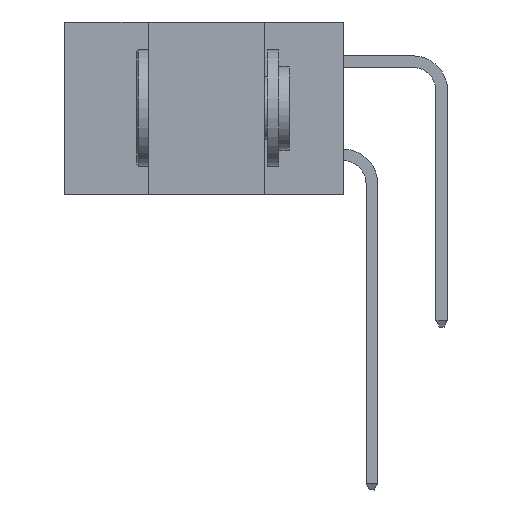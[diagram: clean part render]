
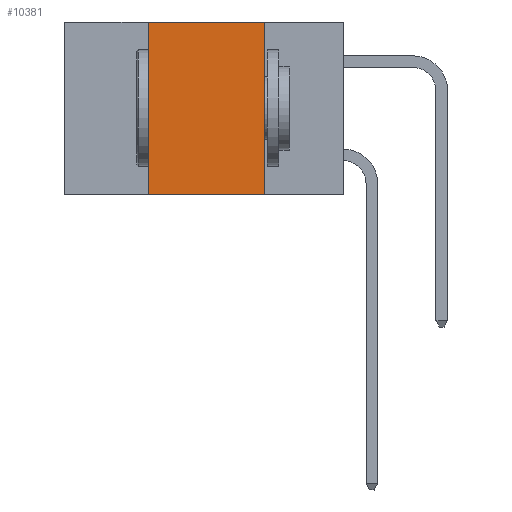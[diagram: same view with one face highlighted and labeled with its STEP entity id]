
A CAD part, left-side view. The second image highlights one B-rep face of the part: STEP entity #10381.
In plain terms, the highlighted planar face has unit normal (-1, 0, 0).
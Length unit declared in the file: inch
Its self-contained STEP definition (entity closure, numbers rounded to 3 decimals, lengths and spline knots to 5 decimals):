
#593 = CARTESIAN_POINT ( 'NONE',  ( 0., 0.17, -0.37 ) ) ;
#629 = ORIENTED_EDGE ( 'NONE', *, *, #6105, .F. ) ;
#1290 = CARTESIAN_POINT ( 'NONE',  ( 0., 0.6, 0. ) ) ;
#1818 = CARTESIAN_POINT ( 'NONE',  ( 0., 0.17, 0. ) ) ;
#2117 = EDGE_CURVE ( 'NONE', #4980, #7276, #3818, .T. ) ;
#2187 = EDGE_LOOP ( 'NONE', ( #10609, #5783, #629, #2998 ) ) ;
#2216 = CARTESIAN_POINT ( 'NONE',  ( 0., 0.6, -0.37 ) ) ;
#2487 = CARTESIAN_POINT ( 'NONE',  ( 0., 0.42, -0.37 ) ) ;
#2998 = ORIENTED_EDGE ( 'NONE', *, *, #4771, .T. ) ;
#3125 = DIRECTION ( 'NONE',  ( 0., -1., 0. ) ) ;
#3818 = LINE ( 'NONE', #5555, #10060 ) ;
#4449 = CARTESIAN_POINT ( 'NONE',  ( 0., 0.42, 0. ) ) ;
#4771 = EDGE_CURVE ( 'NONE', #7574, #7196, #11583, .T. ) ;
#4980 = VERTEX_POINT ( 'NONE', #4449 ) ;
#5460 = DIRECTION ( 'NONE',  ( 0., 0., -1. ) ) ;
#5555 = CARTESIAN_POINT ( 'NONE',  ( 0., 0.6, 0. ) ) ;
#5783 = ORIENTED_EDGE ( 'NONE', *, *, #2117, .F. ) ;
#5823 = AXIS2_PLACEMENT_3D ( 'NONE', #1290, #8947, #11756 ) ;
#5959 = DIRECTION ( 'NONE',  ( 0., 0., 1. ) ) ;
#6105 = EDGE_CURVE ( 'NONE', #7574, #4980, #8616, .T. ) ;
#6467 = VECTOR ( 'NONE', #3125, 39.37008 ) ;
#7196 = VERTEX_POINT ( 'NONE', #7314 ) ;
#7276 = VERTEX_POINT ( 'NONE', #1818 ) ;
#7314 = CARTESIAN_POINT ( 'NONE',  ( 0., 0.17, -0.37 ) ) ;
#7372 = VECTOR ( 'NONE', #5959, 39.37008 ) ;
#7574 = VERTEX_POINT ( 'NONE', #2487 ) ;
#7610 = DIRECTION ( 'NONE',  ( 0., -1., 0. ) ) ;
#7630 = VECTOR ( 'NONE', #5460, 39.37008 ) ;
#7854 = FACE_OUTER_BOUND ( 'NONE', #2187, .T. ) ;
#8616 = LINE ( 'NONE', #9663, #7372 ) ;
#8947 = DIRECTION ( 'NONE',  ( 1., 0., 0. ) ) ;
#9663 = CARTESIAN_POINT ( 'NONE',  ( 0., 0.42, -0.37 ) ) ;
#9815 = PLANE ( 'NONE',  #5823 ) ;
#10060 = VECTOR ( 'NONE', #7610, 39.37008 ) ;
#10381 = ADVANCED_FACE ( 'NONE', ( #7854 ), #9815, .F. ) ;
#10609 = ORIENTED_EDGE ( 'NONE', *, *, #11471, .F. ) ;
#11471 = EDGE_CURVE ( 'NONE', #7276, #7196, #11965, .T. ) ;
#11583 = LINE ( 'NONE', #2216, #6467 ) ;
#11756 = DIRECTION ( 'NONE',  ( 0., 0., -1. ) ) ;
#11965 = LINE ( 'NONE', #593, #7630 ) ;
